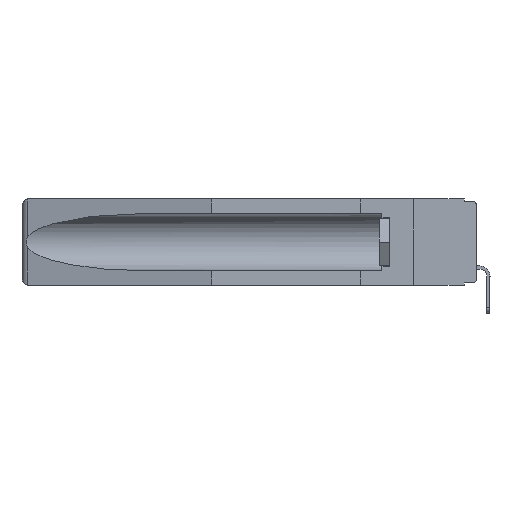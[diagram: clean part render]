
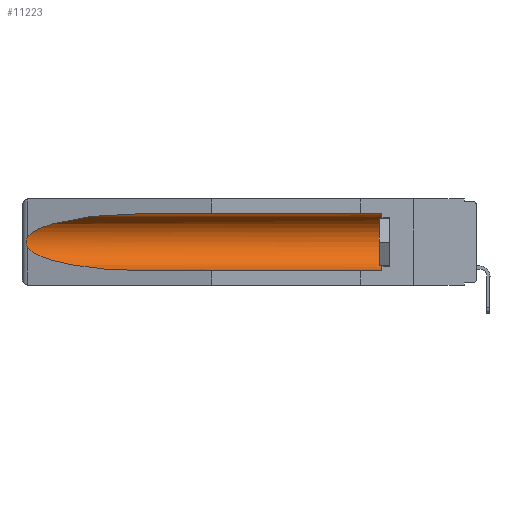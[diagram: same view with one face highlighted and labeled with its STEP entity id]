
A CAD part, left-side view. The second image highlights one B-rep face of the part: STEP entity #11223.
In plain terms, the highlighted cylindrical face has radius 2.857 mm (diameter 5.715 mm), a partial arc.
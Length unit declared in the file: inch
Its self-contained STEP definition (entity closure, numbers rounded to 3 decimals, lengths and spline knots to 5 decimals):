
#433 = DIRECTION ( 'NONE',  ( 0., 1., 0. ) ) ;
#503 = ORIENTED_EDGE ( 'NONE', *, *, #6587, .F. ) ;
#1102 = DIRECTION ( 'NONE',  ( 0., 1., 0. ) ) ;
#1450 = CARTESIAN_POINT ( 'NONE',  ( 0.26537, 1.52718, -0.14972 ) ) ;
#2492 = AXIS2_PLACEMENT_3D ( 'NONE', #17928, #16493, #16579 ) ;
#2826 = ORIENTED_EDGE ( 'NONE', *, *, #8740, .T. ) ;
#3072 = CARTESIAN_POINT ( 'NONE',  ( 0.26654, 1.53092, -0.15636 ) ) ;
#4054 = AXIS2_PLACEMENT_3D ( 'NONE', #7246, #1102, #9815 ) ;
#4125 = CYLINDRICAL_SURFACE ( 'NONE', #4054, 0.1125 ) ;
#4250 = VERTEX_POINT ( 'NONE', #7100 ) ;
#4323 =( BOUNDED_CURVE ( )  B_SPLINE_CURVE ( 3, ( #10724, #9286, #17294, #8608 ),
 .UNSPECIFIED., .F., .F. ) 
 B_SPLINE_CURVE_WITH_KNOTS ( ( 4, 4 ),
 ( 0.1948, 1.5708 ),
 .UNSPECIFIED. ) 
 CURVE ( )  GEOMETRIC_REPRESENTATION_ITEM ( )  RATIONAL_B_SPLINE_CURVE ( ( 1., 0.848, 0.848, 1. ) ) 
 REPRESENTATION_ITEM ( '' )  );
#4818 = VERTEX_POINT ( 'NONE', #4902 ) ;
#4866 = VECTOR ( 'NONE', #8566, 39.37008 ) ;
#4902 = CARTESIAN_POINT ( 'NONE',  ( 0.155, 1.07973, -0.284 ) ) ;
#5178 = EDGE_CURVE ( 'NONE', #8873, #4250, #15960, .T. ) ;
#5387 = CARTESIAN_POINT ( 'NONE',  ( 0.155, 0.126, -0.284 ) ) ;
#5536 = CARTESIAN_POINT ( 'NONE',  ( 0.25451, 1.48313, -0.09465 ) ) ;
#5635 = FACE_OUTER_BOUND ( 'NONE', #15289, .T. ) ;
#6102 = CARTESIAN_POINT ( 'NONE',  ( 0.26655, 1.53094, -0.18657 ) ) ;
#6277 = ORIENTED_EDGE ( 'NONE', *, *, #6823, .T. ) ;
#6587 = EDGE_CURVE ( 'NONE', #17007, #4818, #13430, .T. ) ;
#6823 = EDGE_CURVE ( 'NONE', #12524, #15132, #11611, .T. ) ;
#7100 = CARTESIAN_POINT ( 'NONE',  ( 0.26537, 1.52718, -0.19328 ) ) ;
#7148 = CARTESIAN_POINT ( 'NONE',  ( 0.21114, 1.30732, -0.059 ) ) ;
#7246 = CARTESIAN_POINT ( 'NONE',  ( 0.155, -0.30754, -0.1715 ) ) ;
#7281 = ORIENTED_EDGE ( 'NONE', *, *, #7989, .T. ) ;
#7591 = EDGE_CURVE ( 'NONE', #4250, #4818, #4323, .T. ) ;
#7626 = CARTESIAN_POINT ( 'NONE',  ( 0.26537, 1.52718, -0.19328 ) ) ;
#7652 = CIRCLE ( 'NONE', #2492, 0.1125 ) ;
#7880 = VECTOR ( 'NONE', #433, 39.37008 ) ;
#7989 = EDGE_CURVE ( 'NONE', #15132, #8873, #17824, .T. ) ;
#8566 = DIRECTION ( 'NONE',  ( 0., 1., 0. ) ) ;
#8608 = CARTESIAN_POINT ( 'NONE',  ( 0.155, 1.07973, -0.284 ) ) ;
#8740 = EDGE_CURVE ( 'NONE', #17007, #12524, #7652, .T. ) ;
#8821 = ORIENTED_EDGE ( 'NONE', *, *, #5178, .T. ) ;
#8873 = VERTEX_POINT ( 'NONE', #1450 ) ;
#9286 = CARTESIAN_POINT ( 'NONE',  ( 0.25451, 1.48313, -0.24835 ) ) ;
#9815 = DIRECTION ( 'NONE',  ( 0., 0., 1. ) ) ;
#9904 = CARTESIAN_POINT ( 'NONE',  ( 0.155, 1.07973, -0.059 ) ) ;
#10672 = CARTESIAN_POINT ( 'NONE',  ( 0.2673, 1.5327, -0.16383 ) ) ;
#10724 = CARTESIAN_POINT ( 'NONE',  ( 0.26537, 1.52718, -0.19328 ) ) ;
#11223 = ADVANCED_FACE ( 'NONE', ( #5635 ), #4125, .F. ) ;
#11530 = CARTESIAN_POINT ( 'NONE',  ( 0.26537, 1.52718, -0.14972 ) ) ;
#11611 = LINE ( 'NONE', #13038, #4866 ) ;
#12002 = ORIENTED_EDGE ( 'NONE', *, *, #7591, .T. ) ;
#12524 = VERTEX_POINT ( 'NONE', #14052 ) ;
#13038 = CARTESIAN_POINT ( 'NONE',  ( 0.155, -0.30754, -0.059 ) ) ;
#13040 = CARTESIAN_POINT ( 'NONE',  ( 0.26537, 1.52718, -0.14972 ) ) ;
#13149 = CARTESIAN_POINT ( 'NONE',  ( 0.2673, 1.53269, -0.17917 ) ) ;
#13239 = CARTESIAN_POINT ( 'NONE',  ( 0.26597, 1.52961, -0.15275 ) ) ;
#13330 = CARTESIAN_POINT ( 'NONE',  ( 0.26597, 1.5296, -0.19026 ) ) ;
#13430 = LINE ( 'NONE', #14865, #7880 ) ;
#14052 = CARTESIAN_POINT ( 'NONE',  ( 0.155, 0.126, -0.059 ) ) ;
#14865 = CARTESIAN_POINT ( 'NONE',  ( 0.155, -0.30754, -0.284 ) ) ;
#14958 = CARTESIAN_POINT ( 'NONE',  ( 0.2675, 1.53308, -0.16763 ) ) ;
#15132 = VERTEX_POINT ( 'NONE', #16578 ) ;
#15289 = EDGE_LOOP ( 'NONE', ( #7281, #8821, #12002, #503, #2826, #6277 ) ) ;
#15960 = B_SPLINE_CURVE_WITH_KNOTS ( 'NONE', 3,
 ( #11530, #13239, #3072, #10672, #14958, #17726, #13149, #6102, #13330, #7626 ),
 .UNSPECIFIED., .F., .F.,
 ( 4, 2, 2, 2, 4 ),
 ( 0., 0.00029, 0.00058, 0.00087, 0.00117 ),
 .UNSPECIFIED. ) ;
#16493 = DIRECTION ( 'NONE',  ( 0., -1., 0. ) ) ;
#16578 = CARTESIAN_POINT ( 'NONE',  ( 0.155, 1.07973, -0.059 ) ) ;
#16579 = DIRECTION ( 'NONE',  ( 0., 0., 1. ) ) ;
#17007 = VERTEX_POINT ( 'NONE', #5387 ) ;
#17294 = CARTESIAN_POINT ( 'NONE',  ( 0.21114, 1.30732, -0.284 ) ) ;
#17726 = CARTESIAN_POINT ( 'NONE',  ( 0.2675, 1.53308, -0.17534 ) ) ;
#17824 =( BOUNDED_CURVE ( )  B_SPLINE_CURVE ( 3, ( #9904, #7148, #5536, #13040 ),
 .UNSPECIFIED., .F., .T. ) 
 B_SPLINE_CURVE_WITH_KNOTS ( ( 4, 4 ),
 ( 4.71239, 6.08839 ),
 .UNSPECIFIED. ) 
 CURVE ( )  GEOMETRIC_REPRESENTATION_ITEM ( )  RATIONAL_B_SPLINE_CURVE ( ( 1., 0.848, 0.848, 1. ) ) 
 REPRESENTATION_ITEM ( '' )  );
#17928 = CARTESIAN_POINT ( 'NONE',  ( 0.155, 0.126, -0.1715 ) ) ;
